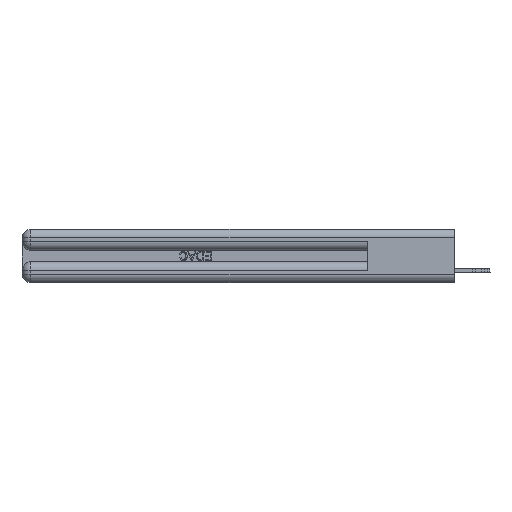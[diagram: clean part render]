
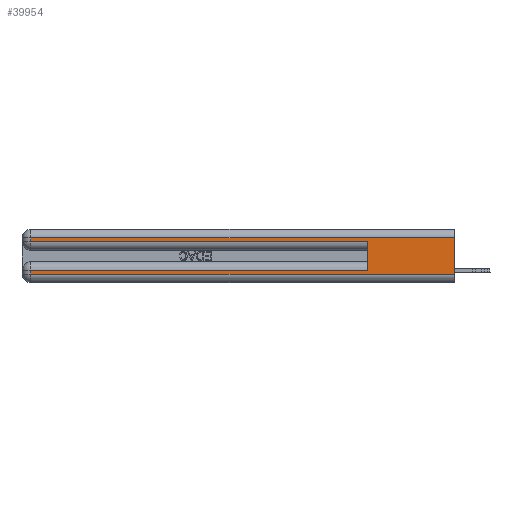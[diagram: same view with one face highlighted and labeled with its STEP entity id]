
A CAD part, left-side view. The second image highlights one B-rep face of the part: STEP entity #39954.
In plain terms, the highlighted planar face has unit normal (-1, 0, 0).
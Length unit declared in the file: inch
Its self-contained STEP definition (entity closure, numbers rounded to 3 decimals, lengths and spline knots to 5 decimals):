
#482 = CARTESIAN_POINT ( 'NONE',  ( 0., 0., 0.37 ) ) ;
#937 = LINE ( 'NONE', #28619, #23528 ) ;
#1963 = VERTEX_POINT ( 'NONE', #7969 ) ;
#3294 = DIRECTION ( 'NONE',  ( 0., -1., 0. ) ) ;
#4751 = DIRECTION ( 'NONE',  ( 0., 0., -1. ) ) ;
#5086 = VERTEX_POINT ( 'NONE', #11769 ) ;
#5142 = CARTESIAN_POINT ( 'NONE',  ( 0., 2.94, 0.085 ) ) ;
#5653 = LINE ( 'NONE', #21891, #38143 ) ;
#5927 = DIRECTION ( 'NONE',  ( 0., 0., -1. ) ) ;
#6953 = EDGE_CURVE ( 'NONE', #1963, #39890, #37739, .T. ) ;
#7702 = CARTESIAN_POINT ( 'NONE',  ( 0., 0., 0.31 ) ) ;
#7969 = CARTESIAN_POINT ( 'NONE',  ( 0., 0.6, 0.085 ) ) ;
#8772 = LINE ( 'NONE', #7702, #50968 ) ;
#9034 = CARTESIAN_POINT ( 'NONE',  ( 0., 0., 0.285 ) ) ;
#9059 = VERTEX_POINT ( 'NONE', #15613 ) ;
#9117 = VERTEX_POINT ( 'NONE', #5142 ) ;
#9877 = ORIENTED_EDGE ( 'NONE', *, *, #39500, .T. ) ;
#11429 = EDGE_CURVE ( 'NONE', #9059, #36413, #8772, .T. ) ;
#11769 = CARTESIAN_POINT ( 'NONE',  ( 0., 2.94, 0.06 ) ) ;
#12523 = EDGE_CURVE ( 'NONE', #21010, #39890, #29817, .T. ) ;
#12981 = DIRECTION ( 'NONE',  ( 1., 0., 0. ) ) ;
#14799 = CARTESIAN_POINT ( 'NONE',  ( 0., 2.94, 0.37 ) ) ;
#15613 = CARTESIAN_POINT ( 'NONE',  ( 0., 0., 0.31 ) ) ;
#15988 = VECTOR ( 'NONE', #40259, 39.37008 ) ;
#16686 = DIRECTION ( 'NONE',  ( 0., 1., 0. ) ) ;
#17355 = PLANE ( 'NONE',  #41641 ) ;
#17708 = EDGE_CURVE ( 'NONE', #36413, #21010, #937, .T. ) ;
#19026 = CARTESIAN_POINT ( 'NONE',  ( 0., 0.6, 0.145 ) ) ;
#19318 = EDGE_LOOP ( 'NONE', ( #39293, #49372, #26480, #24069, #41818, #22218, #9877, #40715 ) ) ;
#21010 = VERTEX_POINT ( 'NONE', #41198 ) ;
#21713 = DIRECTION ( 'NONE',  ( 0., -1., 0. ) ) ;
#21891 = CARTESIAN_POINT ( 'NONE',  ( 0., 0., 0.085 ) ) ;
#22218 = ORIENTED_EDGE ( 'NONE', *, *, #25083, .T. ) ;
#23118 = LINE ( 'NONE', #14799, #15988 ) ;
#23528 = VECTOR ( 'NONE', #5927, 39.37008 ) ;
#24069 = ORIENTED_EDGE ( 'NONE', *, *, #12523, .T. ) ;
#25083 = EDGE_CURVE ( 'NONE', #1963, #9117, #5653, .T. ) ;
#26395 = VECTOR ( 'NONE', #27133, 39.37008 ) ;
#26480 = ORIENTED_EDGE ( 'NONE', *, *, #17708, .T. ) ;
#27133 = DIRECTION ( 'NONE',  ( 0., 0., 1. ) ) ;
#28619 = CARTESIAN_POINT ( 'NONE',  ( 0., 2.94, 0.37 ) ) ;
#29817 = LINE ( 'NONE', #9034, #46373 ) ;
#29970 = EDGE_CURVE ( 'NONE', #9059, #31035, #31389, .T. ) ;
#31035 = VERTEX_POINT ( 'NONE', #49676 ) ;
#31389 = LINE ( 'NONE', #34039, #34096 ) ;
#32868 = EDGE_CURVE ( 'NONE', #5086, #31035, #39141, .T. ) ;
#33207 = FACE_OUTER_BOUND ( 'NONE', #19318, .T. ) ;
#34039 = CARTESIAN_POINT ( 'NONE',  ( 0., 0., 0.37 ) ) ;
#34096 = VECTOR ( 'NONE', #44316, 39.37008 ) ;
#34631 = CARTESIAN_POINT ( 'NONE',  ( 0., 2.94, 0.31 ) ) ;
#36413 = VERTEX_POINT ( 'NONE', #34631 ) ;
#37739 = LINE ( 'NONE', #19026, #26395 ) ;
#38143 = VECTOR ( 'NONE', #51565, 39.37008 ) ;
#39141 = LINE ( 'NONE', #49751, #45132 ) ;
#39293 = ORIENTED_EDGE ( 'NONE', *, *, #29970, .F. ) ;
#39500 = EDGE_CURVE ( 'NONE', #9117, #5086, #23118, .T. ) ;
#39890 = VERTEX_POINT ( 'NONE', #51090 ) ;
#39954 = ADVANCED_FACE ( 'NONE', ( #33207 ), #17355, .F. ) ;
#40259 = DIRECTION ( 'NONE',  ( 0., 0., -1. ) ) ;
#40715 = ORIENTED_EDGE ( 'NONE', *, *, #32868, .T. ) ;
#41198 = CARTESIAN_POINT ( 'NONE',  ( 0., 2.94, 0.285 ) ) ;
#41641 = AXIS2_PLACEMENT_3D ( 'NONE', #482, #12981, #4751 ) ;
#41818 = ORIENTED_EDGE ( 'NONE', *, *, #6953, .F. ) ;
#44316 = DIRECTION ( 'NONE',  ( 0., 0., -1. ) ) ;
#45132 = VECTOR ( 'NONE', #3294, 39.37008 ) ;
#46373 = VECTOR ( 'NONE', #21713, 39.37008 ) ;
#49372 = ORIENTED_EDGE ( 'NONE', *, *, #11429, .T. ) ;
#49676 = CARTESIAN_POINT ( 'NONE',  ( 0., 0., 0.06 ) ) ;
#49751 = CARTESIAN_POINT ( 'NONE',  ( 0., 0., 0.06 ) ) ;
#50968 = VECTOR ( 'NONE', #16686, 39.37008 ) ;
#51090 = CARTESIAN_POINT ( 'NONE',  ( 0., 0.6, 0.285 ) ) ;
#51565 = DIRECTION ( 'NONE',  ( 0., 1., 0. ) ) ;
